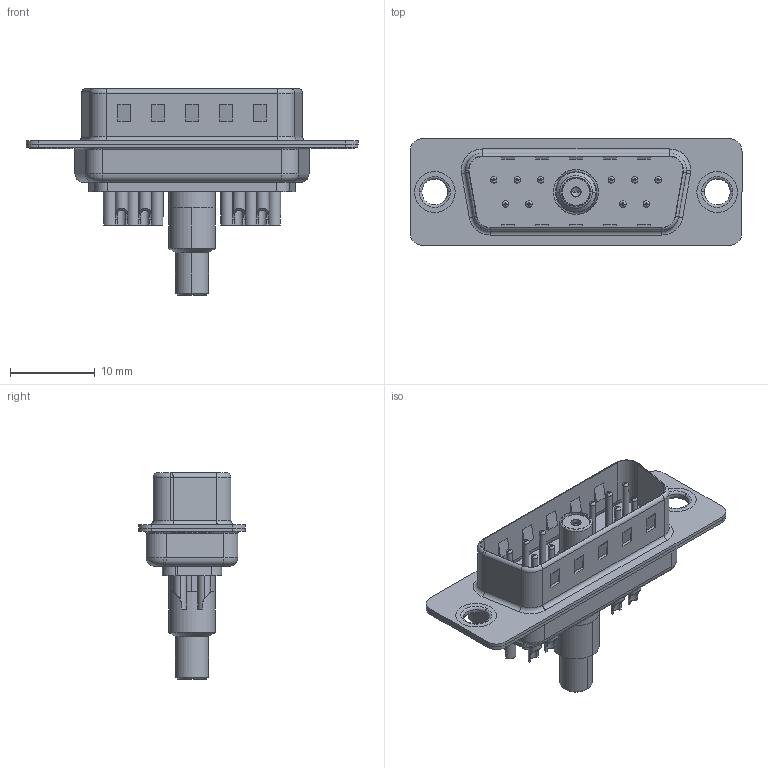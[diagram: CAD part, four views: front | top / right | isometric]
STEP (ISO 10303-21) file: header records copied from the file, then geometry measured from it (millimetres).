
FILE_DESCRIPTION (( 'STEP AP203' ), '1' );
FILE_NAME ('627-11W1622-5N1.STEP', '2019-05-25T14:46:50', ( '' ), ( '' ), 'SwSTEP 2.0', 'SolidWorks 2016', '' );
FILE_SCHEMA (( 'CONFIG_CONTROL_DESIGN' ));
Length unit declared in the file: millimetre
Products named in the file (14): 627-11W1622-5N1; 627Combo Thru Hole Rivet; Co-Ax Jack_Solder Cup Tail; Insulator Socket; Socket_Solder Cup; Insulator Socket 2; Solder Cover; Locking Collar; Co-Ax Jack Assy_SC; 627Combo Housing_11W1; 627Combo Contact Row 1_22; 627Combo Shell Rear_15 Contacts; 627Combo Contact Row 2_22; 627Combo Shell Front_15 Contacts
Assembly tree (22 placements, depth 3):
  627-11W1622-5N1
    627Combo Housing_11W1
    627Combo Shell Rear_15 Contacts
    627Combo Shell Front_15 Contacts
    627Combo Thru Hole Rivet  x2
    Co-Ax Jack Assy_SC
      Co-Ax Jack_Solder Cup Tail
      Insulator Socket
      Insulator Socket 2
      Locking Collar
      Socket_Solder Cup
      Solder Cover
    627Combo Contact Row 1_22  x6
    627Combo Contact Row 2_22  x4
Bounding box: 39.15 x 12.6 x 24.3 mm (x, y, z)
Volume: 1907.3 mm3; surface area: 5559.5 mm2
Topology: 21 solids, 24 shells, 827 faces, 1925 edges, 1182 vertices
Faces by surface type: cylinder 345, plane 278, torus 162, cone 40, bspline 2
Entity records: 18577 total; most frequent: DIRECTION 3127, CARTESIAN_POINT 3055, ORIENTED_EDGE 2694, EDGE_CURVE 1347, AXIS2_PLACEMENT_3D 1230, VERTEX_POINT 846, EDGE_LOOP 685, VECTOR 667
